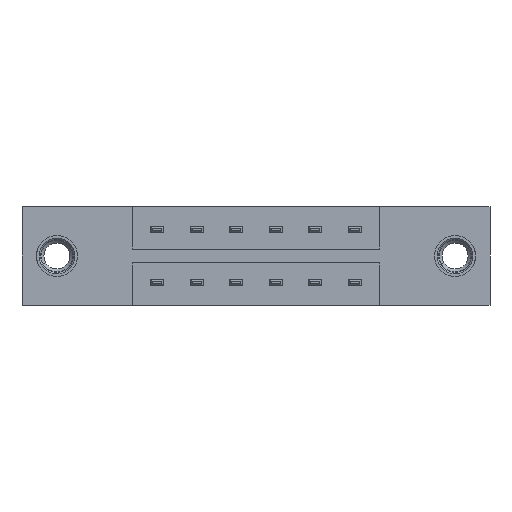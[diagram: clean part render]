
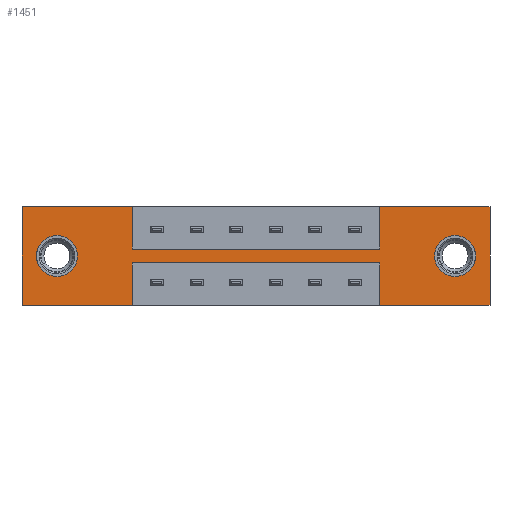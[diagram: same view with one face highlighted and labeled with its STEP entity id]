
A CAD part, front view. The second image highlights one B-rep face of the part: STEP entity #1451.
In plain terms, the highlighted planar face has unit normal (0, -1, 0).
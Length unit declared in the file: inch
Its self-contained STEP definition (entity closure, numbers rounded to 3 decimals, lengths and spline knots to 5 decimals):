
#6 = VECTOR ( 'NONE', #2607, 39.37008 ) ;
#22 = VERTEX_POINT ( 'NONE', #57 ) ;
#53 = DIRECTION ( 'NONE',  ( 0., 1., 0. ) ) ;
#57 = CARTESIAN_POINT ( 'NONE',  ( 1.6425, 0., -0.1095 ) ) ;
#118 = EDGE_CURVE ( 'NONE', #5912, #8458, #3098, .T. ) ;
#121 = VERTEX_POINT ( 'NONE', #8363 ) ;
#291 = CARTESIAN_POINT ( 'NONE',  ( 1.3575, 0., -0.214 ) ) ;
#299 = ORIENTED_EDGE ( 'NONE', *, *, #9216, .F. ) ;
#360 = CARTESIAN_POINT ( 'NONE',  ( 0.4175, 0., -0.161 ) ) ;
#399 = EDGE_CURVE ( 'NONE', #8132, #547, #8759, .T. ) ;
#487 = EDGE_CURVE ( 'NONE', #121, #7713, #5521, .T. ) ;
#505 = ORIENTED_EDGE ( 'NONE', *, *, #487, .T. ) ;
#547 = VERTEX_POINT ( 'NONE', #701 ) ;
#607 = AXIS2_PLACEMENT_3D ( 'NONE', #6384, #8497, #7107 ) ;
#615 = ORIENTED_EDGE ( 'NONE', *, *, #4900, .T. ) ;
#672 = CARTESIAN_POINT ( 'NONE',  ( 1.6425, 0., -0.1875 ) ) ;
#701 = CARTESIAN_POINT ( 'NONE',  ( 0.4175, 0., 0. ) ) ;
#741 = DIRECTION ( 'NONE',  ( 0., 0., -1. ) ) ;
#764 = DIRECTION ( 'NONE',  ( -1., 0., 0. ) ) ;
#802 = CARTESIAN_POINT ( 'NONE',  ( 0.4175, 0., -0.214 ) ) ;
#881 = CARTESIAN_POINT ( 'NONE',  ( 1.775, 0., 0. ) ) ;
#1052 = ORIENTED_EDGE ( 'NONE', *, *, #7283, .F. ) ;
#1199 = PLANE ( 'NONE',  #607 ) ;
#1362 = EDGE_CURVE ( 'NONE', #8764, #8132, #5057, .T. ) ;
#1451 = ADVANCED_FACE ( 'NONE', ( #7451, #6866, #4576 ), #1199, .T. ) ;
#1485 = ORIENTED_EDGE ( 'NONE', *, *, #6435, .F. ) ;
#1570 = CARTESIAN_POINT ( 'NONE',  ( 1.775, 0., 0. ) ) ;
#1905 = CIRCLE ( 'NONE', #8906, 0.078 ) ;
#1985 = ORIENTED_EDGE ( 'NONE', *, *, #118, .F. ) ;
#1996 = DIRECTION ( 'NONE',  ( 1., 0., 0. ) ) ;
#2058 = CARTESIAN_POINT ( 'NONE',  ( 1.775, 0., -0.375 ) ) ;
#2091 = CARTESIAN_POINT ( 'NONE',  ( 0.4175, 0., -0.375 ) ) ;
#2162 = EDGE_CURVE ( 'NONE', #3344, #8403, #7160, .T. ) ;
#2199 = VERTEX_POINT ( 'NONE', #2751 ) ;
#2207 = VERTEX_POINT ( 'NONE', #8664 ) ;
#2238 = ORIENTED_EDGE ( 'NONE', *, *, #6930, .F. ) ;
#2254 = DIRECTION ( 'NONE',  ( 0., 0., -1. ) ) ;
#2281 = DIRECTION ( 'NONE',  ( 0., 0., 1. ) ) ;
#2607 = DIRECTION ( 'NONE',  ( -1., 0., 0. ) ) ;
#2674 = VECTOR ( 'NONE', #6139, 39.37008 ) ;
#2731 = ORIENTED_EDGE ( 'NONE', *, *, #7771, .F. ) ;
#2746 = ORIENTED_EDGE ( 'NONE', *, *, #4146, .F. ) ;
#2751 = CARTESIAN_POINT ( 'NONE',  ( 1.3575, 0., -0.214 ) ) ;
#2849 = AXIS2_PLACEMENT_3D ( 'NONE', #7485, #3881, #8230 ) ;
#2863 = LINE ( 'NONE', #8055, #7575 ) ;
#2898 = EDGE_CURVE ( 'NONE', #6120, #8764, #8181, .T. ) ;
#2960 = AXIS2_PLACEMENT_3D ( 'NONE', #5902, #8052, #4309 ) ;
#3039 = CARTESIAN_POINT ( 'NONE',  ( 0.1325, 0., -0.1875 ) ) ;
#3098 = LINE ( 'NONE', #9023, #3321 ) ;
#3221 = EDGE_LOOP ( 'NONE', ( #4325, #505 ) ) ;
#3321 = VECTOR ( 'NONE', #6851, 39.37008 ) ;
#3344 = VERTEX_POINT ( 'NONE', #8601 ) ;
#3471 = VECTOR ( 'NONE', #3782, 39.37008 ) ;
#3535 = CARTESIAN_POINT ( 'NONE',  ( 0., 0., 0. ) ) ;
#3701 = ORIENTED_EDGE ( 'NONE', *, *, #1362, .F. ) ;
#3775 = EDGE_CURVE ( 'NONE', #7214, #2207, #2863, .T. ) ;
#3782 = DIRECTION ( 'NONE',  ( 0., 0., 1. ) ) ;
#3843 = EDGE_CURVE ( 'NONE', #7713, #121, #1905, .T. ) ;
#3881 = DIRECTION ( 'NONE',  ( 0., 1., 0. ) ) ;
#4021 = LINE ( 'NONE', #7080, #6 ) ;
#4080 = ORIENTED_EDGE ( 'NONE', *, *, #2162, .F. ) ;
#4113 = ORIENTED_EDGE ( 'NONE', *, *, #399, .F. ) ;
#4146 = EDGE_CURVE ( 'NONE', #547, #7214, #6552, .T. ) ;
#4223 = CARTESIAN_POINT ( 'NONE',  ( 0., 0., 0. ) ) ;
#4309 = DIRECTION ( 'NONE',  ( 0., 0., 1. ) ) ;
#4325 = ORIENTED_EDGE ( 'NONE', *, *, #3843, .T. ) ;
#4352 = CARTESIAN_POINT ( 'NONE',  ( 0., 0., -0.375 ) ) ;
#4372 = VECTOR ( 'NONE', #764, 39.37008 ) ;
#4386 = CIRCLE ( 'NONE', #5016, 0.078 ) ;
#4540 = ORIENTED_EDGE ( 'NONE', *, *, #2898, .F. ) ;
#4576 = FACE_OUTER_BOUND ( 'NONE', #8699, .T. ) ;
#4900 = EDGE_CURVE ( 'NONE', #22, #7489, #8261, .T. ) ;
#4981 = DIRECTION ( 'NONE',  ( 1., 0., 0. ) ) ;
#5016 = AXIS2_PLACEMENT_3D ( 'NONE', #672, #53, #741 ) ;
#5057 = LINE ( 'NONE', #6943, #6767 ) ;
#5073 = VECTOR ( 'NONE', #4981, 39.37008 ) ;
#5118 = VECTOR ( 'NONE', #2254, 39.37008 ) ;
#5177 = CARTESIAN_POINT ( 'NONE',  ( 0.1325, 0., -0.1095 ) ) ;
#5264 = DIRECTION ( 'NONE',  ( 0., 0., -1. ) ) ;
#5521 = CIRCLE ( 'NONE', #2960, 0.078 ) ;
#5548 = VECTOR ( 'NONE', #1996, 39.37008 ) ;
#5788 = LINE ( 'NONE', #6653, #3471 ) ;
#5902 = CARTESIAN_POINT ( 'NONE',  ( 0.1325, 0., -0.1875 ) ) ;
#5912 = VERTEX_POINT ( 'NONE', #2058 ) ;
#6120 = VERTEX_POINT ( 'NONE', #2091 ) ;
#6139 = DIRECTION ( 'NONE',  ( 0., 0., 1. ) ) ;
#6147 = DIRECTION ( 'NONE',  ( 0., 0., 1. ) ) ;
#6272 = VECTOR ( 'NONE', #5264, 39.37008 ) ;
#6307 = CARTESIAN_POINT ( 'NONE',  ( 1.6425, 0., -0.2655 ) ) ;
#6384 = CARTESIAN_POINT ( 'NONE',  ( 0., 0., -0.375 ) ) ;
#6435 = EDGE_CURVE ( 'NONE', #9048, #6120, #8217, .T. ) ;
#6445 = DIRECTION ( 'NONE',  ( 0., 0., -1. ) ) ;
#6552 = LINE ( 'NONE', #8326, #8270 ) ;
#6653 = CARTESIAN_POINT ( 'NONE',  ( 1.3575, 0., -0.161 ) ) ;
#6767 = VECTOR ( 'NONE', #6147, 39.37008 ) ;
#6824 = LINE ( 'NONE', #291, #2674 ) ;
#6851 = DIRECTION ( 'NONE',  ( -1., 0., 0. ) ) ;
#6866 = FACE_BOUND ( 'NONE', #3221, .T. ) ;
#6930 = EDGE_CURVE ( 'NONE', #8403, #5912, #7394, .T. ) ;
#6943 = CARTESIAN_POINT ( 'NONE',  ( 0., 0., 0. ) ) ;
#7080 = CARTESIAN_POINT ( 'NONE',  ( 0.4175, 0., -0.214 ) ) ;
#7103 = CARTESIAN_POINT ( 'NONE',  ( 0., 0., 0. ) ) ;
#7107 = DIRECTION ( 'NONE',  ( 0., 0., -1. ) ) ;
#7160 = LINE ( 'NONE', #7103, #5548 ) ;
#7214 = VERTEX_POINT ( 'NONE', #360 ) ;
#7283 = EDGE_CURVE ( 'NONE', #8458, #2199, #6824, .T. ) ;
#7394 = LINE ( 'NONE', #881, #5118 ) ;
#7451 = FACE_BOUND ( 'NONE', #7716, .T. ) ;
#7485 = CARTESIAN_POINT ( 'NONE',  ( 1.6425, 0., -0.1875 ) ) ;
#7489 = VERTEX_POINT ( 'NONE', #6307 ) ;
#7517 = DIRECTION ( 'NONE',  ( 0., 1., 0. ) ) ;
#7575 = VECTOR ( 'NONE', #8113, 39.37008 ) ;
#7679 = CARTESIAN_POINT ( 'NONE',  ( 1.3575, 0., -0.375 ) ) ;
#7713 = VERTEX_POINT ( 'NONE', #5177 ) ;
#7716 = EDGE_LOOP ( 'NONE', ( #615, #8624 ) ) ;
#7771 = EDGE_CURVE ( 'NONE', #2207, #3344, #5788, .T. ) ;
#7897 = CARTESIAN_POINT ( 'NONE',  ( 0., 0., -0.375 ) ) ;
#7957 = ORIENTED_EDGE ( 'NONE', *, *, #3775, .F. ) ;
#8052 = DIRECTION ( 'NONE',  ( 0., 1., 0. ) ) ;
#8055 = CARTESIAN_POINT ( 'NONE',  ( 0.4175, 0., -0.161 ) ) ;
#8113 = DIRECTION ( 'NONE',  ( 1., 0., 0. ) ) ;
#8132 = VERTEX_POINT ( 'NONE', #3535 ) ;
#8164 = EDGE_CURVE ( 'NONE', #7489, #22, #4386, .T. ) ;
#8181 = LINE ( 'NONE', #4352, #4372 ) ;
#8217 = LINE ( 'NONE', #8315, #6272 ) ;
#8230 = DIRECTION ( 'NONE',  ( 0., 0., -1. ) ) ;
#8261 = CIRCLE ( 'NONE', #2849, 0.078 ) ;
#8270 = VECTOR ( 'NONE', #6445, 39.37008 ) ;
#8315 = CARTESIAN_POINT ( 'NONE',  ( 0.4175, 0., -0.214 ) ) ;
#8326 = CARTESIAN_POINT ( 'NONE',  ( 0.4175, 0., -0.161 ) ) ;
#8363 = CARTESIAN_POINT ( 'NONE',  ( 0.1325, 0., -0.2655 ) ) ;
#8403 = VERTEX_POINT ( 'NONE', #1570 ) ;
#8458 = VERTEX_POINT ( 'NONE', #7679 ) ;
#8497 = DIRECTION ( 'NONE',  ( 0., -1., 0. ) ) ;
#8601 = CARTESIAN_POINT ( 'NONE',  ( 1.3575, 0., 0. ) ) ;
#8624 = ORIENTED_EDGE ( 'NONE', *, *, #8164, .T. ) ;
#8664 = CARTESIAN_POINT ( 'NONE',  ( 1.3575, 0., -0.161 ) ) ;
#8699 = EDGE_LOOP ( 'NONE', ( #1052, #1985, #2238, #4080, #2731, #7957, #2746, #4113, #3701, #4540, #1485, #299 ) ) ;
#8759 = LINE ( 'NONE', #4223, #5073 ) ;
#8764 = VERTEX_POINT ( 'NONE', #7897 ) ;
#8906 = AXIS2_PLACEMENT_3D ( 'NONE', #3039, #7517, #2281 ) ;
#9023 = CARTESIAN_POINT ( 'NONE',  ( 0., 0., -0.375 ) ) ;
#9048 = VERTEX_POINT ( 'NONE', #802 ) ;
#9216 = EDGE_CURVE ( 'NONE', #2199, #9048, #4021, .T. ) ;
